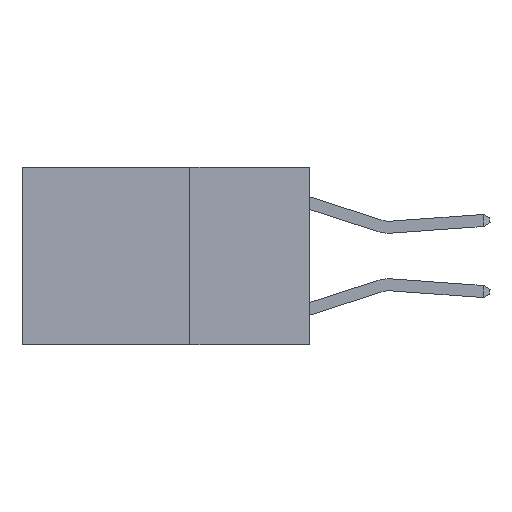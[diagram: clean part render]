
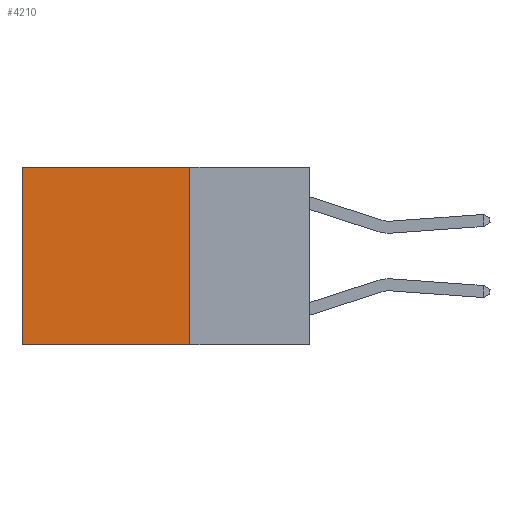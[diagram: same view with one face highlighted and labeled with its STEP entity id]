
A CAD part, left-side view. The second image highlights one B-rep face of the part: STEP entity #4210.
In plain terms, the highlighted planar face has unit normal (-1, 0, 0).
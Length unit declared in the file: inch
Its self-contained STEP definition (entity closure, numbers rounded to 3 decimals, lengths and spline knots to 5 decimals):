
#409 = EDGE_CURVE ( 'NONE', #5050, #17821, #7103, .T. ) ;
#1618 = ORIENTED_EDGE ( 'NONE', *, *, #9707, .F. ) ;
#2878 = DIRECTION ( 'NONE',  ( 0., 0., -1. ) ) ;
#3286 = CARTESIAN_POINT ( 'NONE',  ( 0.2625, 0.6, -0.37 ) ) ;
#4137 = CARTESIAN_POINT ( 'NONE',  ( 0.2625, 0.25, 0. ) ) ;
#4210 = ADVANCED_FACE ( 'NONE', ( #15305 ), #5056, .F. ) ;
#4730 = CARTESIAN_POINT ( 'NONE',  ( 0.2625, 0.25, -0.37 ) ) ;
#5050 = VERTEX_POINT ( 'NONE', #12448 ) ;
#5056 = PLANE ( 'NONE',  #19129 ) ;
#5216 = VERTEX_POINT ( 'NONE', #4730 ) ;
#5766 = CARTESIAN_POINT ( 'NONE',  ( 0.2625, 0.25, 0. ) ) ;
#6370 = CARTESIAN_POINT ( 'NONE',  ( 0.2625, 0.6, 0. ) ) ;
#6632 = CARTESIAN_POINT ( 'NONE',  ( 0.2625, 0.6, 0. ) ) ;
#6648 = ORIENTED_EDGE ( 'NONE', *, *, #14466, .F. ) ;
#7103 = LINE ( 'NONE', #4137, #20127 ) ;
#8559 = DIRECTION ( 'NONE',  ( 0., 1., 0. ) ) ;
#9075 = CARTESIAN_POINT ( 'NONE',  ( 0.2625, 0.25, -0.37 ) ) ;
#9137 = LINE ( 'NONE', #5766, #17638 ) ;
#9537 = LINE ( 'NONE', #6370, #20788 ) ;
#9707 = EDGE_CURVE ( 'NONE', #5216, #18787, #16300, .T. ) ;
#10285 = ORIENTED_EDGE ( 'NONE', *, *, #20033, .T. ) ;
#11927 = DIRECTION ( 'NONE',  ( 1., 0., 0. ) ) ;
#12448 = CARTESIAN_POINT ( 'NONE',  ( 0.2625, 0.25, 0. ) ) ;
#12645 = DIRECTION ( 'NONE',  ( 0., 0., -1. ) ) ;
#14466 = EDGE_CURVE ( 'NONE', #5050, #5216, #9137, .T. ) ;
#14474 = DIRECTION ( 'NONE',  ( 0., 1., 0. ) ) ;
#15305 = FACE_OUTER_BOUND ( 'NONE', #20530, .T. ) ;
#15326 = ORIENTED_EDGE ( 'NONE', *, *, #409, .T. ) ;
#15958 = VECTOR ( 'NONE', #14474, 39.37008 ) ;
#16300 = LINE ( 'NONE', #9075, #15958 ) ;
#17638 = VECTOR ( 'NONE', #12645, 39.37008 ) ;
#17821 = VERTEX_POINT ( 'NONE', #6632 ) ;
#18787 = VERTEX_POINT ( 'NONE', #3286 ) ;
#19129 = AXIS2_PLACEMENT_3D ( 'NONE', #20157, #11927, #20598 ) ;
#20033 = EDGE_CURVE ( 'NONE', #17821, #18787, #9537, .T. ) ;
#20127 = VECTOR ( 'NONE', #8559, 39.37008 ) ;
#20157 = CARTESIAN_POINT ( 'NONE',  ( 0.2625, 0.25, 0. ) ) ;
#20530 = EDGE_LOOP ( 'NONE', ( #10285, #1618, #6648, #15326 ) ) ;
#20598 = DIRECTION ( 'NONE',  ( 0., 0., -1. ) ) ;
#20788 = VECTOR ( 'NONE', #2878, 39.37008 ) ;
